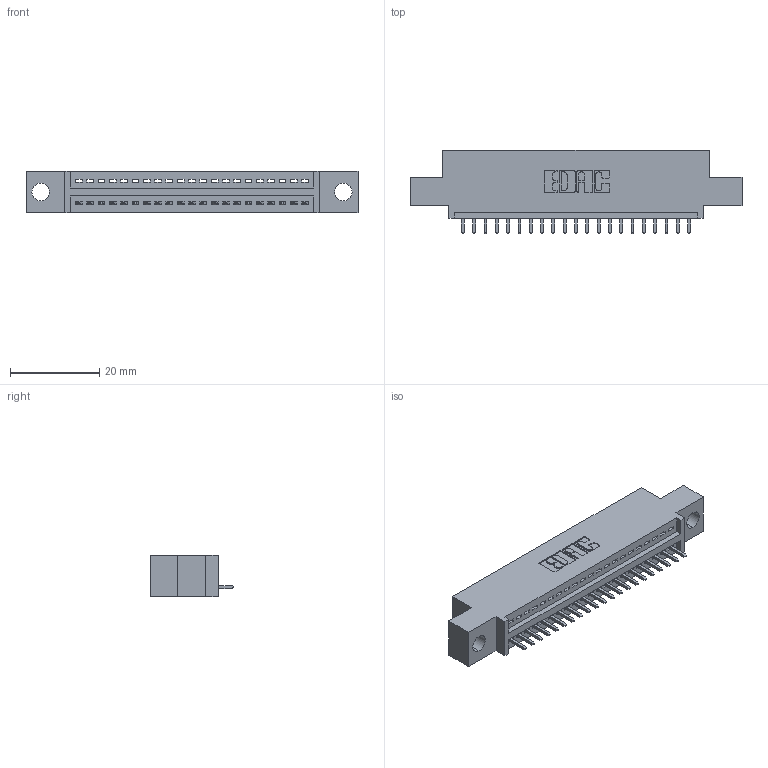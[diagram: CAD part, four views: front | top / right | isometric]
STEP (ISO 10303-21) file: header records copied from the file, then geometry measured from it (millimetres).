
FILE_DESCRIPTION (( 'STEP AP203' ), '1' );
FILE_NAME ('395-021-521-404.STEP', '2021-05-31T14:29:50', ( '' ), ( '' ), 'SwSTEP 2.0', 'SolidWorks 2020', '' );
FILE_SCHEMA (( 'CONFIG_CONTROL_DESIGN' ));
Length unit declared in the file: inch
Products named in the file (3): 395-021-521-404; 345 Part_0.110 Offset - 0.156 Dia-TI; 345-292-001_345-293-121
Assembly tree (22 placements, depth 2):
  395-021-521-404
    345 Part_0.110 Offset - 0.156 Dia-TI
    345-292-001_345-293-121  x21
Bounding box: 74.55 x 18.72 x 9.4 mm (x, y, z)
Volume: 6669.7 mm3; surface area: 8268.6 mm2
Topology: 22 solids, 22 shells, 1362 faces, 4085 edges, 2694 vertices
Faces by surface type: plane 938, cylinder 424
Entity records: 19201 total; most frequent: CARTESIAN_POINT 3337, ORIENTED_EDGE 3290, DIRECTION 2943, EDGE_CURVE 1645, LINE 1429, VECTOR 1429, VERTEX_POINT 1094, AXIS2_PLACEMENT_3D 757
